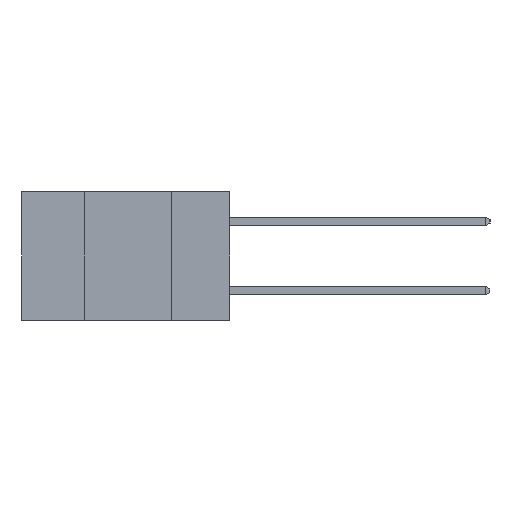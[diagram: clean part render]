
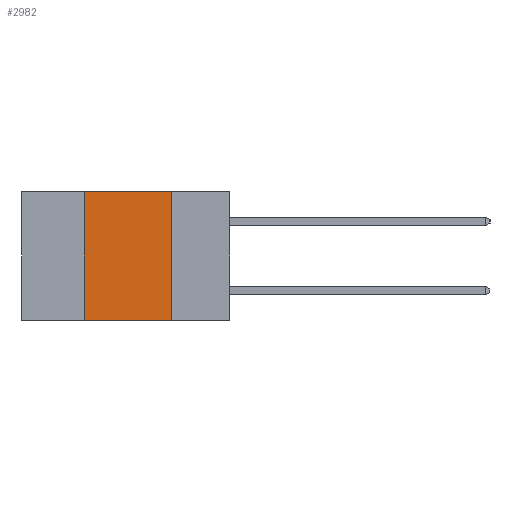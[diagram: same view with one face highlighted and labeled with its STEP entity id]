
A CAD part, left-side view. The second image highlights one B-rep face of the part: STEP entity #2982.
In plain terms, the highlighted planar face has unit normal (-1, 0, 0).
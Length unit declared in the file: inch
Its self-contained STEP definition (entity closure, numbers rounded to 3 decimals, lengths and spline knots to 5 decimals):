
#193 = EDGE_CURVE ( 'NONE', #15744, #2125, #13807, .T. ) ;
#574 = EDGE_LOOP ( 'NONE', ( #13468, #18119, #624, #5259 ) ) ;
#624 = ORIENTED_EDGE ( 'NONE', *, *, #193, .F. ) ;
#885 = VERTEX_POINT ( 'NONE', #20038 ) ;
#899 = CARTESIAN_POINT ( 'NONE',  ( 0., 0.17, 0. ) ) ;
#2125 = VERTEX_POINT ( 'NONE', #7636 ) ;
#2430 = CARTESIAN_POINT ( 'NONE',  ( 0., 0.42, -0.37 ) ) ;
#2982 = ADVANCED_FACE ( 'NONE', ( #3856 ), #19035, .F. ) ;
#3697 = EDGE_CURVE ( 'NONE', #2125, #7747, #12293, .T. ) ;
#3856 = FACE_OUTER_BOUND ( 'NONE', #574, .T. ) ;
#4185 = AXIS2_PLACEMENT_3D ( 'NONE', #18475, #17914, #17795 ) ;
#4579 = DIRECTION ( 'NONE',  ( 0., 0., -1. ) ) ;
#5145 = DIRECTION ( 'NONE',  ( 0., 0., 1. ) ) ;
#5259 = ORIENTED_EDGE ( 'NONE', *, *, #21658, .T. ) ;
#7168 = EDGE_CURVE ( 'NONE', #7747, #885, #14138, .T. ) ;
#7636 = CARTESIAN_POINT ( 'NONE',  ( 0., 0.42, 0. ) ) ;
#7747 = VERTEX_POINT ( 'NONE', #899 ) ;
#9596 = CARTESIAN_POINT ( 'NONE',  ( 0., 0.42, -0.37 ) ) ;
#9680 = VECTOR ( 'NONE', #5145, 39.37008 ) ;
#9705 = VECTOR ( 'NONE', #18770, 39.37008 ) ;
#12293 = LINE ( 'NONE', #21674, #21552 ) ;
#13287 = CARTESIAN_POINT ( 'NONE',  ( 0., 0.17, -0.37 ) ) ;
#13468 = ORIENTED_EDGE ( 'NONE', *, *, #7168, .F. ) ;
#13807 = LINE ( 'NONE', #2430, #9680 ) ;
#14138 = LINE ( 'NONE', #13287, #21736 ) ;
#15744 = VERTEX_POINT ( 'NONE', #9596 ) ;
#16991 = CARTESIAN_POINT ( 'NONE',  ( 0., 0.6, -0.37 ) ) ;
#17795 = DIRECTION ( 'NONE',  ( 0., 0., -1. ) ) ;
#17914 = DIRECTION ( 'NONE',  ( 1., 0., 0. ) ) ;
#18119 = ORIENTED_EDGE ( 'NONE', *, *, #3697, .F. ) ;
#18475 = CARTESIAN_POINT ( 'NONE',  ( 0., 0.6, 0. ) ) ;
#18770 = DIRECTION ( 'NONE',  ( 0., -1., 0. ) ) ;
#19035 = PLANE ( 'NONE',  #4185 ) ;
#19043 = LINE ( 'NONE', #16991, #9705 ) ;
#20038 = CARTESIAN_POINT ( 'NONE',  ( 0., 0.17, -0.37 ) ) ;
#21552 = VECTOR ( 'NONE', #21783, 39.37008 ) ;
#21658 = EDGE_CURVE ( 'NONE', #15744, #885, #19043, .T. ) ;
#21674 = CARTESIAN_POINT ( 'NONE',  ( 0., 0.6, 0. ) ) ;
#21736 = VECTOR ( 'NONE', #4579, 39.37008 ) ;
#21783 = DIRECTION ( 'NONE',  ( 0., -1., 0. ) ) ;
